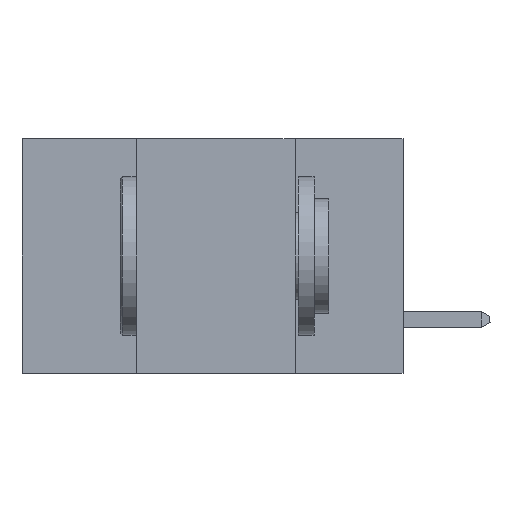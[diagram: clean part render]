
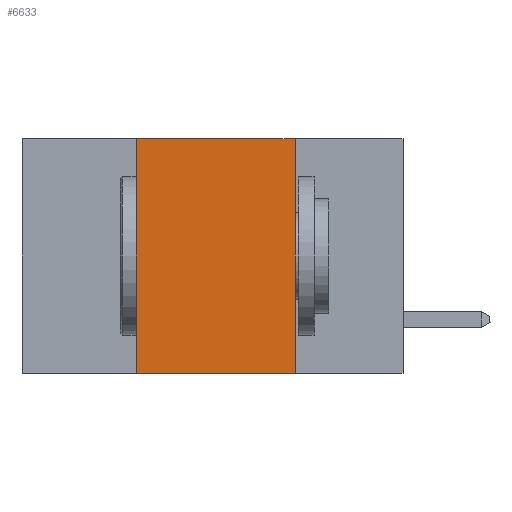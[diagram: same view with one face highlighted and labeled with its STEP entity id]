
A CAD part, left-side view. The second image highlights one B-rep face of the part: STEP entity #6633.
In plain terms, the highlighted planar face has unit normal (-1, 0, 0).
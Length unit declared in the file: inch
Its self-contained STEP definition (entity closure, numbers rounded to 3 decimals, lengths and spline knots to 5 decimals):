
#10 = DIRECTION ( 'NONE',  ( 0., 0., -1. ) ) ;
#720 = FACE_OUTER_BOUND ( 'NONE', #4285, .T. ) ;
#725 = EDGE_CURVE ( 'NONE', #11706, #19996, #17207, .T. ) ;
#1569 = EDGE_CURVE ( 'NONE', #19996, #12479, #18700, .T. ) ;
#2702 = DIRECTION ( 'NONE',  ( 0., 0., -1. ) ) ;
#2725 = CARTESIAN_POINT ( 'NONE',  ( 0., 0.6, -0.37 ) ) ;
#3948 = ORIENTED_EDGE ( 'NONE', *, *, #725, .F. ) ;
#4285 = EDGE_LOOP ( 'NONE', ( #19392, #3948, #15612, #7283 ) ) ;
#4649 = EDGE_CURVE ( 'NONE', #9591, #11706, #19289, .T. ) ;
#5803 = DIRECTION ( 'NONE',  ( 1., 0., 0. ) ) ;
#5891 = CARTESIAN_POINT ( 'NONE',  ( 0., 0.17, -0.37 ) ) ;
#5905 = CARTESIAN_POINT ( 'NONE',  ( 0., 0.6, 0. ) ) ;
#6118 = VECTOR ( 'NONE', #17149, 39.37008 ) ;
#6561 = DIRECTION ( 'NONE',  ( 0., 0., 1. ) ) ;
#6633 = ADVANCED_FACE ( 'NONE', ( #720 ), #9056, .F. ) ;
#7184 = VECTOR ( 'NONE', #10, 39.37008 ) ;
#7283 = ORIENTED_EDGE ( 'NONE', *, *, #10512, .T. ) ;
#7418 = CARTESIAN_POINT ( 'NONE',  ( 0., 0.6, 0. ) ) ;
#8850 = CARTESIAN_POINT ( 'NONE',  ( 0., 0.42, 0. ) ) ;
#9056 = PLANE ( 'NONE',  #18022 ) ;
#9591 = VERTEX_POINT ( 'NONE', #12015 ) ;
#10512 = EDGE_CURVE ( 'NONE', #9591, #12479, #17355, .T. ) ;
#10992 = CARTESIAN_POINT ( 'NONE',  ( 0., 0.17, 0. ) ) ;
#11141 = CARTESIAN_POINT ( 'NONE',  ( 0., 0.17, 0. ) ) ;
#11706 = VERTEX_POINT ( 'NONE', #8850 ) ;
#12015 = CARTESIAN_POINT ( 'NONE',  ( 0., 0.42, -0.37 ) ) ;
#12479 = VERTEX_POINT ( 'NONE', #5891 ) ;
#14223 = VECTOR ( 'NONE', #15422, 39.37008 ) ;
#14413 = CARTESIAN_POINT ( 'NONE',  ( 0., 0.42, 0. ) ) ;
#15059 = VECTOR ( 'NONE', #6561, 39.37008 ) ;
#15422 = DIRECTION ( 'NONE',  ( 0., -1., 0. ) ) ;
#15612 = ORIENTED_EDGE ( 'NONE', *, *, #4649, .F. ) ;
#17149 = DIRECTION ( 'NONE',  ( 0., -1., 0. ) ) ;
#17207 = LINE ( 'NONE', #5905, #14223 ) ;
#17355 = LINE ( 'NONE', #2725, #6118 ) ;
#18022 = AXIS2_PLACEMENT_3D ( 'NONE', #7418, #5803, #2702 ) ;
#18700 = LINE ( 'NONE', #11141, #7184 ) ;
#19289 = LINE ( 'NONE', #14413, #15059 ) ;
#19392 = ORIENTED_EDGE ( 'NONE', *, *, #1569, .F. ) ;
#19996 = VERTEX_POINT ( 'NONE', #10992 ) ;
